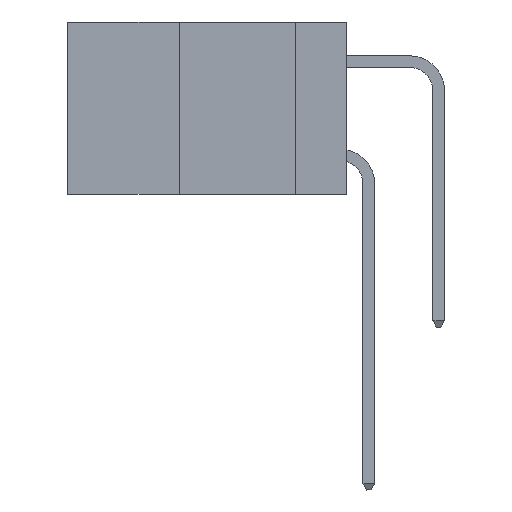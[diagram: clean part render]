
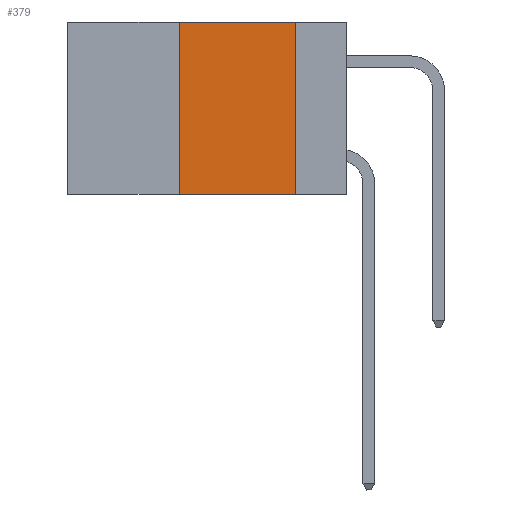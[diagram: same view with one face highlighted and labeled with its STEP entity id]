
A CAD part, left-side view. The second image highlights one B-rep face of the part: STEP entity #379.
In plain terms, the highlighted planar face has unit normal (-1, 0, 0).
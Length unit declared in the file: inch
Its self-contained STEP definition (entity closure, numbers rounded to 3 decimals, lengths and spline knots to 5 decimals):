
#379 = ADVANCED_FACE ( 'NONE', ( #11211 ), #14052, .F. ) ;
#2321 = CARTESIAN_POINT ( 'NONE',  ( 0., 0.36, 0. ) ) ;
#3757 = AXIS2_PLACEMENT_3D ( 'NONE', #16979, #5190, #17107 ) ;
#3921 = CARTESIAN_POINT ( 'NONE',  ( 0., 0.6, -0.37 ) ) ;
#4779 = DIRECTION ( 'NONE',  ( 0., 0., -1. ) ) ;
#4861 = EDGE_CURVE ( 'NONE', #9517, #15038, #13785, .T. ) ;
#4941 = VERTEX_POINT ( 'NONE', #2321 ) ;
#5143 = CARTESIAN_POINT ( 'NONE',  ( 0., 0.36, 0. ) ) ;
#5190 = DIRECTION ( 'NONE',  ( 1., 0., 0. ) ) ;
#5547 = LINE ( 'NONE', #11528, #6891 ) ;
#6502 = VECTOR ( 'NONE', #4779, 39.37008 ) ;
#6891 = VECTOR ( 'NONE', #7367, 39.37008 ) ;
#6931 = EDGE_CURVE ( 'NONE', #9517, #4941, #8339, .T. ) ;
#7367 = DIRECTION ( 'NONE',  ( 0., -1., 0. ) ) ;
#7380 = EDGE_CURVE ( 'NONE', #7476, #15038, #14883, .T. ) ;
#7476 = VERTEX_POINT ( 'NONE', #9968 ) ;
#7654 = CARTESIAN_POINT ( 'NONE',  ( 0., 0.11, 0. ) ) ;
#8339 = LINE ( 'NONE', #5143, #16670 ) ;
#9517 = VERTEX_POINT ( 'NONE', #13682 ) ;
#9968 = CARTESIAN_POINT ( 'NONE',  ( 0., 0.11, 0. ) ) ;
#10945 = ORIENTED_EDGE ( 'NONE', *, *, #6931, .F. ) ;
#11211 = FACE_OUTER_BOUND ( 'NONE', #14628, .T. ) ;
#11528 = CARTESIAN_POINT ( 'NONE',  ( 0., 0.6, 0. ) ) ;
#11905 = CARTESIAN_POINT ( 'NONE',  ( 0., 0.11, -0.37 ) ) ;
#12423 = ORIENTED_EDGE ( 'NONE', *, *, #7380, .F. ) ;
#13682 = CARTESIAN_POINT ( 'NONE',  ( 0., 0.36, -0.37 ) ) ;
#13785 = LINE ( 'NONE', #3921, #19089 ) ;
#14052 = PLANE ( 'NONE',  #3757 ) ;
#14628 = EDGE_LOOP ( 'NONE', ( #12423, #17461, #10945, #15611 ) ) ;
#14883 = LINE ( 'NONE', #7654, #6502 ) ;
#15038 = VERTEX_POINT ( 'NONE', #11905 ) ;
#15611 = ORIENTED_EDGE ( 'NONE', *, *, #4861, .T. ) ;
#16670 = VECTOR ( 'NONE', #18306, 39.37008 ) ;
#16808 = EDGE_CURVE ( 'NONE', #4941, #7476, #5547, .T. ) ;
#16979 = CARTESIAN_POINT ( 'NONE',  ( 0., 0.6, 0. ) ) ;
#16999 = DIRECTION ( 'NONE',  ( 0., -1., 0. ) ) ;
#17107 = DIRECTION ( 'NONE',  ( 0., 0., -1. ) ) ;
#17461 = ORIENTED_EDGE ( 'NONE', *, *, #16808, .F. ) ;
#18306 = DIRECTION ( 'NONE',  ( 0., 0., 1. ) ) ;
#19089 = VECTOR ( 'NONE', #16999, 39.37008 ) ;
